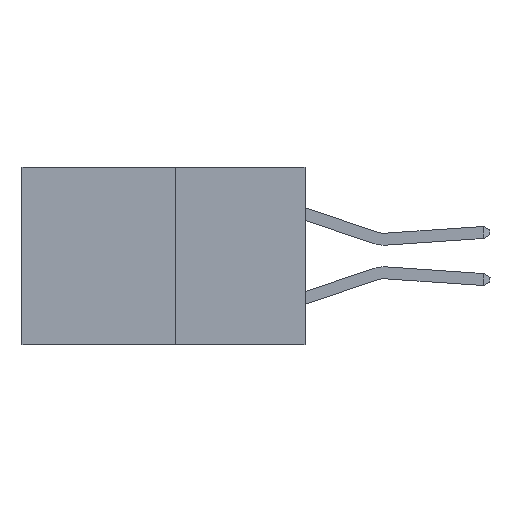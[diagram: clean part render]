
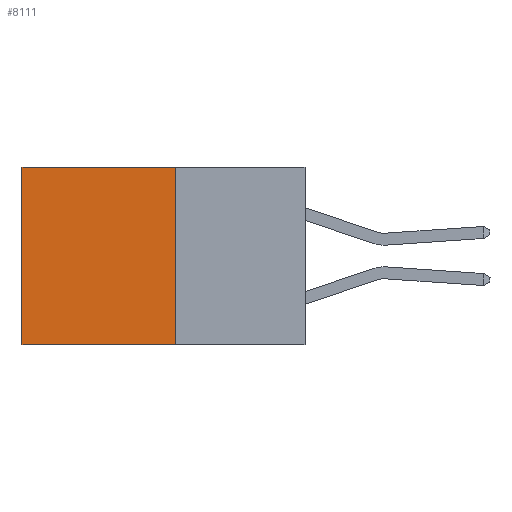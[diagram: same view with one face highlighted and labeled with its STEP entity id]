
A CAD part, left-side view. The second image highlights one B-rep face of the part: STEP entity #8111.
In plain terms, the highlighted planar face has unit normal (-1, 0, 0).
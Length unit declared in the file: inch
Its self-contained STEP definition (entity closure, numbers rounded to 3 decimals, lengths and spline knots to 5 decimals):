
#200 = ORIENTED_EDGE ( 'NONE', *, *, #12474, .T. ) ;
#203 = VECTOR ( 'NONE', #12058, 39.37008 ) ;
#364 = VECTOR ( 'NONE', #2874, 39.37008 ) ;
#408 = VERTEX_POINT ( 'NONE', #7896 ) ;
#825 = CARTESIAN_POINT ( 'NONE',  ( 0.277, 0.59, -0.37 ) ) ;
#941 = CARTESIAN_POINT ( 'NONE',  ( 0.277, 0.27, -0.37 ) ) ;
#946 = EDGE_CURVE ( 'NONE', #1344, #1639, #1775, .T. ) ;
#1344 = VERTEX_POINT ( 'NONE', #3132 ) ;
#1639 = VERTEX_POINT ( 'NONE', #9128 ) ;
#1754 = EDGE_CURVE ( 'NONE', #408, #1344, #10431, .T. ) ;
#1775 = LINE ( 'NONE', #941, #11586 ) ;
#2874 = DIRECTION ( 'NONE',  ( 0., 0., -1. ) ) ;
#3132 = CARTESIAN_POINT ( 'NONE',  ( 0.277, 0.27, -0.37 ) ) ;
#4035 = VERTEX_POINT ( 'NONE', #4541 ) ;
#4175 = DIRECTION ( 'NONE',  ( 1., 0., 0. ) ) ;
#4541 = CARTESIAN_POINT ( 'NONE',  ( 0.277, 0.59, 0. ) ) ;
#5489 = AXIS2_PLACEMENT_3D ( 'NONE', #7979, #4175, #10987 ) ;
#6009 = CARTESIAN_POINT ( 'NONE',  ( 0.277, 0.27, -0.37 ) ) ;
#6405 = CARTESIAN_POINT ( 'NONE',  ( 0.277, 0.27, 0. ) ) ;
#6762 = DIRECTION ( 'NONE',  ( 0., 0., -1. ) ) ;
#7896 = CARTESIAN_POINT ( 'NONE',  ( 0.277, 0.27, 0. ) ) ;
#7930 = LINE ( 'NONE', #6405, #203 ) ;
#7979 = CARTESIAN_POINT ( 'NONE',  ( 0.277, 0.27, -0.37 ) ) ;
#8105 = DIRECTION ( 'NONE',  ( 0., 1., 0. ) ) ;
#8111 = ADVANCED_FACE ( 'NONE', ( #9530 ), #10065, .F. ) ;
#9128 = CARTESIAN_POINT ( 'NONE',  ( 0.277, 0.59, -0.37 ) ) ;
#9530 = FACE_OUTER_BOUND ( 'NONE', #10837, .T. ) ;
#9857 = ORIENTED_EDGE ( 'NONE', *, *, #12150, .T. ) ;
#10065 = PLANE ( 'NONE',  #5489 ) ;
#10142 = VECTOR ( 'NONE', #6762, 39.37008 ) ;
#10152 = ORIENTED_EDGE ( 'NONE', *, *, #946, .F. ) ;
#10431 = LINE ( 'NONE', #6009, #10142 ) ;
#10837 = EDGE_LOOP ( 'NONE', ( #9857, #10152, #12547, #200 ) ) ;
#10877 = LINE ( 'NONE', #825, #364 ) ;
#10987 = DIRECTION ( 'NONE',  ( 0., 0., -1. ) ) ;
#11586 = VECTOR ( 'NONE', #8105, 39.37008 ) ;
#12058 = DIRECTION ( 'NONE',  ( 0., 1., 0. ) ) ;
#12150 = EDGE_CURVE ( 'NONE', #4035, #1639, #10877, .T. ) ;
#12474 = EDGE_CURVE ( 'NONE', #408, #4035, #7930, .T. ) ;
#12547 = ORIENTED_EDGE ( 'NONE', *, *, #1754, .F. ) ;
